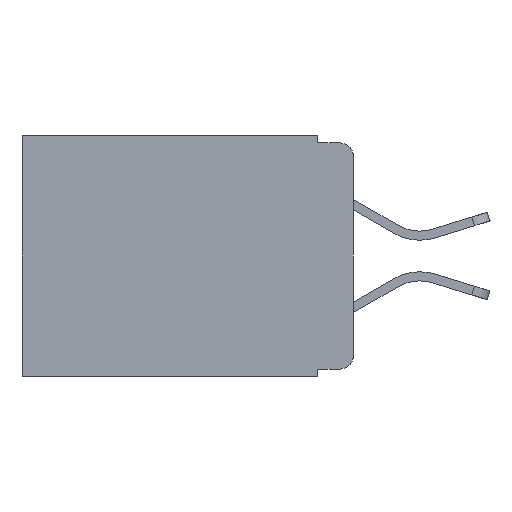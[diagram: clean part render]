
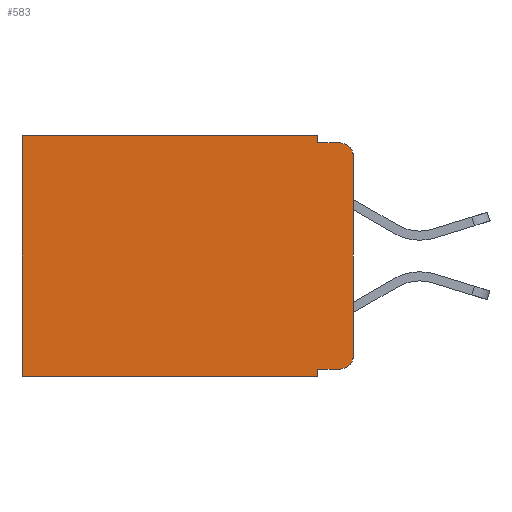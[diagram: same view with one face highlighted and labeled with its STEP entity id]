
A CAD part, left-side view. The second image highlights one B-rep face of the part: STEP entity #583.
In plain terms, the highlighted planar face has unit normal (-1, 0, 0).
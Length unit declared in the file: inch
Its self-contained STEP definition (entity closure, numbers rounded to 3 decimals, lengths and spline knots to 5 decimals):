
#84 = EDGE_CURVE ( 'NONE', #6097, #271, #12602, .T. ) ;
#216 = CARTESIAN_POINT ( 'NONE',  ( 0.298, 0.051, -0.333 ) ) ;
#271 = VERTEX_POINT ( 'NONE', #2717 ) ;
#407 = PLANE ( 'NONE',  #1653 ) ;
#477 = EDGE_CURVE ( 'NONE', #3319, #7141, #5140, .T. ) ;
#583 = ADVANCED_FACE ( 'NONE', ( #8188 ), #407, .F. ) ;
#627 = CARTESIAN_POINT ( 'NONE',  ( 0.298, 0.473, 0. ) ) ;
#1355 = DIRECTION ( 'NONE',  ( 0., 0., -1. ) ) ;
#1404 = AXIS2_PLACEMENT_3D ( 'NONE', #2497, #9657, #3688 ) ;
#1653 = AXIS2_PLACEMENT_3D ( 'NONE', #7912, #9874, #1355 ) ;
#1808 = DIRECTION ( 'NONE',  ( 0., 0., -1. ) ) ;
#1854 = ORIENTED_EDGE ( 'NONE', *, *, #84, .F. ) ;
#2143 = VERTEX_POINT ( 'NONE', #12693 ) ;
#2420 = CARTESIAN_POINT ( 'NONE',  ( 0.298, 0., -0.343 ) ) ;
#2479 = DIRECTION ( 'NONE',  ( 0., 0., -1. ) ) ;
#2497 = CARTESIAN_POINT ( 'NONE',  ( 0.298, 0.02, -0.313 ) ) ;
#2717 = CARTESIAN_POINT ( 'NONE',  ( 0.298, 0., -0.313 ) ) ;
#2895 = LINE ( 'NONE', #5741, #12819 ) ;
#3319 = VERTEX_POINT ( 'NONE', #3898 ) ;
#3504 = DIRECTION ( 'NONE',  ( -1., 0., 0. ) ) ;
#3688 = DIRECTION ( 'NONE',  ( 0., 0., -1. ) ) ;
#3898 = CARTESIAN_POINT ( 'NONE',  ( 0.298, 0.051, -0.343 ) ) ;
#3921 = AXIS2_PLACEMENT_3D ( 'NONE', #9539, #3504, #10412 ) ;
#4139 = ORIENTED_EDGE ( 'NONE', *, *, #9561, .T. ) ;
#4348 = LINE ( 'NONE', #12925, #9833 ) ;
#4612 = ORIENTED_EDGE ( 'NONE', *, *, #477, .F. ) ;
#4632 = DIRECTION ( 'NONE',  ( 0., 1., 0. ) ) ;
#5140 = LINE ( 'NONE', #2420, #7414 ) ;
#5189 = ORIENTED_EDGE ( 'NONE', *, *, #8997, .F. ) ;
#5245 = DIRECTION ( 'NONE',  ( 0., 1., 0. ) ) ;
#5376 = VECTOR ( 'NONE', #6946, 39.37008 ) ;
#5687 = CARTESIAN_POINT ( 'NONE',  ( 0.298, 0.473, 0. ) ) ;
#5741 = CARTESIAN_POINT ( 'NONE',  ( 0.298, 0., 0. ) ) ;
#5746 = ORIENTED_EDGE ( 'NONE', *, *, #7348, .T. ) ;
#5809 = CARTESIAN_POINT ( 'NONE',  ( 0.298, 0.051, -0.333 ) ) ;
#6046 = LINE ( 'NONE', #627, #10936 ) ;
#6097 = VERTEX_POINT ( 'NONE', #11164 ) ;
#6531 = CARTESIAN_POINT ( 'NONE',  ( 0.298, 0.051, -0.01 ) ) ;
#6577 = LINE ( 'NONE', #7674, #9407 ) ;
#6946 = DIRECTION ( 'NONE',  ( 0., -1., 0. ) ) ;
#7141 = VERTEX_POINT ( 'NONE', #9538 ) ;
#7204 = CARTESIAN_POINT ( 'NONE',  ( 0.298, 0.051, 0. ) ) ;
#7232 = EDGE_CURVE ( 'NONE', #10108, #3319, #6577, .T. ) ;
#7348 = EDGE_CURVE ( 'NONE', #10108, #10987, #12908, .T. ) ;
#7414 = VECTOR ( 'NONE', #5245, 39.37008 ) ;
#7505 = EDGE_LOOP ( 'NONE', ( #1854, #10317, #12162, #5189, #8682, #4139, #4612, #10301, #5746, #10959 ) ) ;
#7592 = DIRECTION ( 'NONE',  ( 0., -1., 0. ) ) ;
#7674 = CARTESIAN_POINT ( 'NONE',  ( 0.298, 0.051, 0. ) ) ;
#7890 = VECTOR ( 'NONE', #11612, 39.37008 ) ;
#7912 = CARTESIAN_POINT ( 'NONE',  ( 0.298, 0., 0. ) ) ;
#7930 = EDGE_CURVE ( 'NONE', #10987, #271, #11428, .T. ) ;
#8164 = CARTESIAN_POINT ( 'NONE',  ( 0.298, 0., 0. ) ) ;
#8188 = FACE_OUTER_BOUND ( 'NONE', #7505, .T. ) ;
#8192 = DIRECTION ( 'NONE',  ( 0., 0., -1. ) ) ;
#8682 = ORIENTED_EDGE ( 'NONE', *, *, #9339, .T. ) ;
#8997 = EDGE_CURVE ( 'NONE', #12588, #12402, #11265, .T. ) ;
#9339 = EDGE_CURVE ( 'NONE', #12588, #12519, #2895, .T. ) ;
#9407 = VECTOR ( 'NONE', #2479, 39.37008 ) ;
#9538 = CARTESIAN_POINT ( 'NONE',  ( 0.298, 0.473, -0.343 ) ) ;
#9539 = CARTESIAN_POINT ( 'NONE',  ( 0.298, 0.02, -0.03 ) ) ;
#9561 = EDGE_CURVE ( 'NONE', #12519, #7141, #6046, .T. ) ;
#9571 = CIRCLE ( 'NONE', #3921, 0.02 ) ;
#9657 = DIRECTION ( 'NONE',  ( -1., 0., 0. ) ) ;
#9833 = VECTOR ( 'NONE', #7592, 39.37008 ) ;
#9874 = DIRECTION ( 'NONE',  ( 1., 0., 0. ) ) ;
#10108 = VERTEX_POINT ( 'NONE', #5809 ) ;
#10189 = CARTESIAN_POINT ( 'NONE',  ( 0.298, 0.02, -0.333 ) ) ;
#10301 = ORIENTED_EDGE ( 'NONE', *, *, #7232, .F. ) ;
#10317 = ORIENTED_EDGE ( 'NONE', *, *, #11329, .T. ) ;
#10412 = DIRECTION ( 'NONE',  ( 0., 0., -1. ) ) ;
#10936 = VECTOR ( 'NONE', #8192, 39.37008 ) ;
#10959 = ORIENTED_EDGE ( 'NONE', *, *, #7930, .T. ) ;
#10987 = VERTEX_POINT ( 'NONE', #10189 ) ;
#11003 = VECTOR ( 'NONE', #1808, 39.37008 ) ;
#11164 = CARTESIAN_POINT ( 'NONE',  ( 0.298, 0., -0.03 ) ) ;
#11239 = CARTESIAN_POINT ( 'NONE',  ( 0.298, 0.051, 0. ) ) ;
#11258 = EDGE_CURVE ( 'NONE', #12402, #2143, #4348, .T. ) ;
#11265 = LINE ( 'NONE', #7204, #11003 ) ;
#11329 = EDGE_CURVE ( 'NONE', #6097, #2143, #9571, .T. ) ;
#11428 = CIRCLE ( 'NONE', #1404, 0.02 ) ;
#11612 = DIRECTION ( 'NONE',  ( 0., 0., -1. ) ) ;
#12162 = ORIENTED_EDGE ( 'NONE', *, *, #11258, .F. ) ;
#12402 = VERTEX_POINT ( 'NONE', #6531 ) ;
#12519 = VERTEX_POINT ( 'NONE', #5687 ) ;
#12588 = VERTEX_POINT ( 'NONE', #11239 ) ;
#12602 = LINE ( 'NONE', #8164, #7890 ) ;
#12693 = CARTESIAN_POINT ( 'NONE',  ( 0.298, 0.02, -0.01 ) ) ;
#12819 = VECTOR ( 'NONE', #4632, 39.37008 ) ;
#12908 = LINE ( 'NONE', #216, #5376 ) ;
#12925 = CARTESIAN_POINT ( 'NONE',  ( 0.298, 0.051, -0.01 ) ) ;
